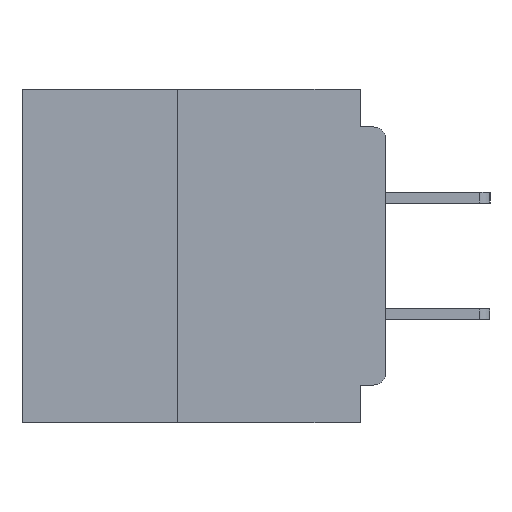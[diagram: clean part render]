
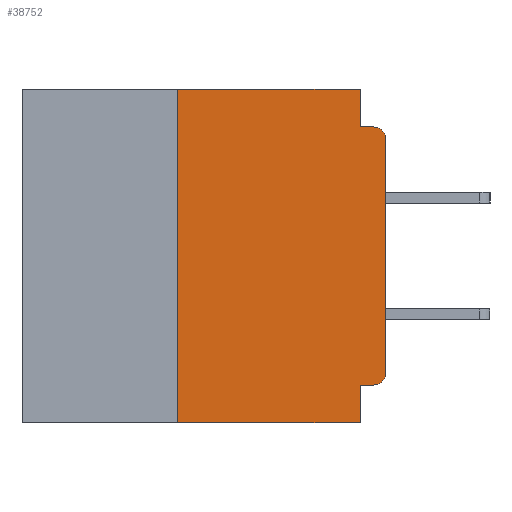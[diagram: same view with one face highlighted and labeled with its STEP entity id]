
A CAD part, left-side view. The second image highlights one B-rep face of the part: STEP entity #38752.
In plain terms, the highlighted planar face has unit normal (-1, 0, 0).
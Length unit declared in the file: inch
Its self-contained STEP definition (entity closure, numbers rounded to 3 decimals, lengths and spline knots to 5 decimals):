
#733 = PLANE ( 'NONE',  #4606 ) ;
#1085 = VERTEX_POINT ( 'NONE', #14228 ) ;
#3617 = CARTESIAN_POINT ( 'NONE',  ( 0., 0.25, -0.4 ) ) ;
#3897 = DIRECTION ( 'NONE',  ( 0., 0., -1. ) ) ;
#4136 = CARTESIAN_POINT ( 'NONE',  ( 0., 0., -0.06 ) ) ;
#4606 = AXIS2_PLACEMENT_3D ( 'NONE', #28918, #4804, #32959 ) ;
#4804 = DIRECTION ( 'NONE',  ( 1., 0., 0. ) ) ;
#5443 = CARTESIAN_POINT ( 'NONE',  ( 0., 0.25, -0.4 ) ) ;
#5810 = LINE ( 'NONE', #19131, #48473 ) ;
#6204 = VECTOR ( 'NONE', #48065, 39.37008 ) ;
#6914 = CARTESIAN_POINT ( 'NONE',  ( 0., 0.031, -0.355 ) ) ;
#7549 = CARTESIAN_POINT ( 'NONE',  ( 0., 0., -0.34 ) ) ;
#8274 = AXIS2_PLACEMENT_3D ( 'NONE', #17772, #45711, #21815 ) ;
#9750 = CARTESIAN_POINT ( 'NONE',  ( 0., 0.031, -0.4 ) ) ;
#10300 = DIRECTION ( 'NONE',  ( -1., 0., 0. ) ) ;
#11156 = CARTESIAN_POINT ( 'NONE',  ( 0., 0.437, -0.4 ) ) ;
#12197 = ORIENTED_EDGE ( 'NONE', *, *, #44821, .T. ) ;
#12294 = AXIS2_PLACEMENT_3D ( 'NONE', #34353, #10300, #38360 ) ;
#12447 = CARTESIAN_POINT ( 'NONE',  ( 0., 0.015, -0.355 ) ) ;
#12525 = VERTEX_POINT ( 'NONE', #18275 ) ;
#13207 = VERTEX_POINT ( 'NONE', #13680 ) ;
#13312 = CARTESIAN_POINT ( 'NONE',  ( 0., 0., -0.355 ) ) ;
#13417 = EDGE_CURVE ( 'NONE', #34287, #13207, #5810, .T. ) ;
#13680 = CARTESIAN_POINT ( 'NONE',  ( 0., 0.031, 0. ) ) ;
#14228 = CARTESIAN_POINT ( 'NONE',  ( 0., 0.031, -0.045 ) ) ;
#16123 = EDGE_CURVE ( 'NONE', #50303, #39219, #48877, .T. ) ;
#16474 = ORIENTED_EDGE ( 'NONE', *, *, #21138, .F. ) ;
#17659 = VECTOR ( 'NONE', #37658, 39.37008 ) ;
#17772 = CARTESIAN_POINT ( 'NONE',  ( 0., 0.015, -0.06 ) ) ;
#17848 = VECTOR ( 'NONE', #35768, 39.37008 ) ;
#18275 = CARTESIAN_POINT ( 'NONE',  ( 0., 0.015, -0.045 ) ) ;
#19131 = CARTESIAN_POINT ( 'NONE',  ( 0., 0.437, 0. ) ) ;
#20275 = CIRCLE ( 'NONE', #12294, 0.015 ) ;
#20903 = FACE_OUTER_BOUND ( 'NONE', #27072, .T. ) ;
#21138 = EDGE_CURVE ( 'NONE', #51357, #34287, #39129, .T. ) ;
#21370 = EDGE_CURVE ( 'NONE', #44544, #49619, #30371, .T. ) ;
#21675 = ORIENTED_EDGE ( 'NONE', *, *, #41645, .T. ) ;
#21815 = DIRECTION ( 'NONE',  ( 0., 0., -1. ) ) ;
#22061 = ORIENTED_EDGE ( 'NONE', *, *, #45962, .T. ) ;
#23542 = DIRECTION ( 'NONE',  ( 0., 0., -1. ) ) ;
#24009 = CARTESIAN_POINT ( 'NONE',  ( 0., 0.031, -0.4 ) ) ;
#24563 = ORIENTED_EDGE ( 'NONE', *, *, #27699, .F. ) ;
#27072 = EDGE_LOOP ( 'NONE', ( #34867, #22061, #43263, #24563, #49028, #16474, #21675, #40073, #43621, #12197 ) ) ;
#27317 = DIRECTION ( 'NONE',  ( 0., -1., 0. ) ) ;
#27656 = CIRCLE ( 'NONE', #8274, 0.015 ) ;
#27699 = EDGE_CURVE ( 'NONE', #13207, #1085, #49302, .T. ) ;
#28918 = CARTESIAN_POINT ( 'NONE',  ( 0., 0.437, 0. ) ) ;
#30371 = LINE ( 'NONE', #13312, #49122 ) ;
#32959 = DIRECTION ( 'NONE',  ( 0., 0., -1. ) ) ;
#34287 = VERTEX_POINT ( 'NONE', #46406 ) ;
#34353 = CARTESIAN_POINT ( 'NONE',  ( 0., 0.015, -0.34 ) ) ;
#34834 = VERTEX_POINT ( 'NONE', #9750 ) ;
#34867 = ORIENTED_EDGE ( 'NONE', *, *, #16123, .T. ) ;
#35429 = CARTESIAN_POINT ( 'NONE',  ( 0., 0.031, 0. ) ) ;
#35768 = DIRECTION ( 'NONE',  ( 0., 0., 1. ) ) ;
#37402 = VECTOR ( 'NONE', #23542, 39.37008 ) ;
#37658 = DIRECTION ( 'NONE',  ( 0., -1., 0. ) ) ;
#38360 = DIRECTION ( 'NONE',  ( 0., 0., -1. ) ) ;
#38680 = VECTOR ( 'NONE', #27317, 39.37008 ) ;
#38752 = ADVANCED_FACE ( 'NONE', ( #20903 ), #733, .F. ) ;
#38937 = LINE ( 'NONE', #45497, #17659 ) ;
#39129 = LINE ( 'NONE', #3617, #17848 ) ;
#39219 = VERTEX_POINT ( 'NONE', #4136 ) ;
#39440 = EDGE_CURVE ( 'NONE', #1085, #12525, #38937, .T. ) ;
#40073 = ORIENTED_EDGE ( 'NONE', *, *, #45058, .F. ) ;
#41333 = DIRECTION ( 'NONE',  ( 0., 1., 0. ) ) ;
#41645 = EDGE_CURVE ( 'NONE', #51357, #34834, #49330, .T. ) ;
#43263 = ORIENTED_EDGE ( 'NONE', *, *, #39440, .F. ) ;
#43621 = ORIENTED_EDGE ( 'NONE', *, *, #21370, .F. ) ;
#44544 = VERTEX_POINT ( 'NONE', #12447 ) ;
#44821 = EDGE_CURVE ( 'NONE', #44544, #50303, #20275, .T. ) ;
#45058 = EDGE_CURVE ( 'NONE', #49619, #34834, #51498, .T. ) ;
#45497 = CARTESIAN_POINT ( 'NONE',  ( 0., 0., -0.045 ) ) ;
#45711 = DIRECTION ( 'NONE',  ( -1., 0., 0. ) ) ;
#45962 = EDGE_CURVE ( 'NONE', #39219, #12525, #27656, .T. ) ;
#46406 = CARTESIAN_POINT ( 'NONE',  ( 0., 0.25, 0. ) ) ;
#47097 = DIRECTION ( 'NONE',  ( 0., -1., 0. ) ) ;
#48065 = DIRECTION ( 'NONE',  ( 0., 0., 1. ) ) ;
#48244 = CARTESIAN_POINT ( 'NONE',  ( 0., 0., 0. ) ) ;
#48473 = VECTOR ( 'NONE', #47097, 39.37008 ) ;
#48877 = LINE ( 'NONE', #48244, #6204 ) ;
#49028 = ORIENTED_EDGE ( 'NONE', *, *, #13417, .F. ) ;
#49122 = VECTOR ( 'NONE', #41333, 39.37008 ) ;
#49302 = LINE ( 'NONE', #35429, #37402 ) ;
#49330 = LINE ( 'NONE', #11156, #38680 ) ;
#49619 = VERTEX_POINT ( 'NONE', #6914 ) ;
#50256 = VECTOR ( 'NONE', #3897, 39.37008 ) ;
#50303 = VERTEX_POINT ( 'NONE', #7549 ) ;
#51357 = VERTEX_POINT ( 'NONE', #5443 ) ;
#51498 = LINE ( 'NONE', #24009, #50256 ) ;
